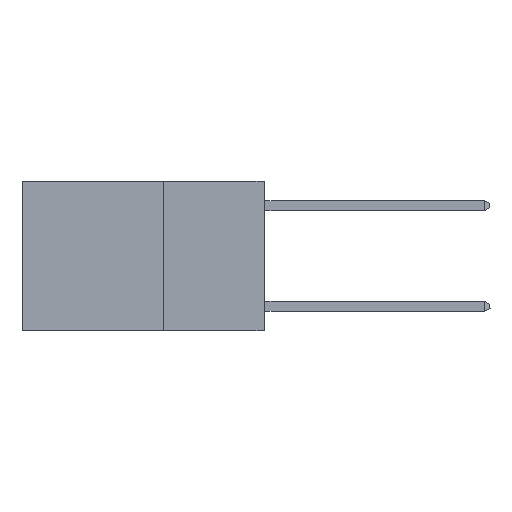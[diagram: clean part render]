
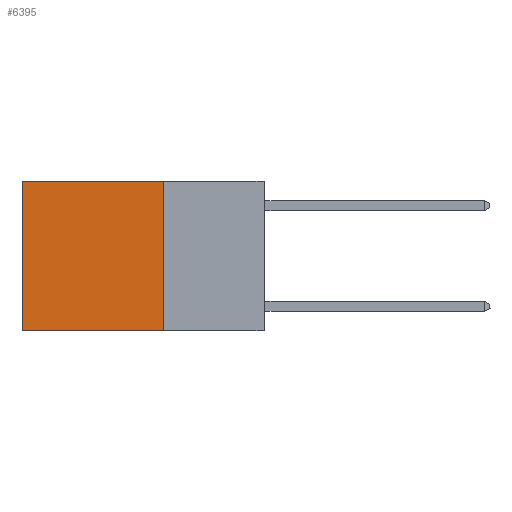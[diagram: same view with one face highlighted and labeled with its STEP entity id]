
A CAD part, left-side view. The second image highlights one B-rep face of the part: STEP entity #6395.
In plain terms, the highlighted planar face has unit normal (-1, 0, 0).
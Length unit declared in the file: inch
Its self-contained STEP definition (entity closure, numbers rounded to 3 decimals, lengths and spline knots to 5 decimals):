
#464 = CARTESIAN_POINT ( 'NONE',  ( 0.2625, 0.25, -0.37 ) ) ;
#875 = PLANE ( 'NONE',  #8818 ) ;
#888 = CARTESIAN_POINT ( 'NONE',  ( 0.2625, 0.25, -0.37 ) ) ;
#2189 = VERTEX_POINT ( 'NONE', #6380 ) ;
#2240 = DIRECTION ( 'NONE',  ( 1., 0., 0. ) ) ;
#2431 = CARTESIAN_POINT ( 'NONE',  ( 0.2625, 0.25, 0. ) ) ;
#2490 = LINE ( 'NONE', #888, #2856 ) ;
#2638 = CARTESIAN_POINT ( 'NONE',  ( 0.2625, 0.25, 0. ) ) ;
#2707 = CARTESIAN_POINT ( 'NONE',  ( 0.2625, 0.25, 0. ) ) ;
#2856 = VECTOR ( 'NONE', #7996, 39.37008 ) ;
#3342 = VERTEX_POINT ( 'NONE', #464 ) ;
#3536 = EDGE_CURVE ( 'NONE', #11224, #3342, #7976, .T. ) ;
#3630 = EDGE_LOOP ( 'NONE', ( #8910, #8903, #8497, #6399 ) ) ;
#4560 = EDGE_CURVE ( 'NONE', #11224, #5095, #10932, .T. ) ;
#4590 = DIRECTION ( 'NONE',  ( 0., 1., 0. ) ) ;
#5095 = VERTEX_POINT ( 'NONE', #8430 ) ;
#5472 = EDGE_CURVE ( 'NONE', #5095, #2189, #7646, .T. ) ;
#5748 = EDGE_CURVE ( 'NONE', #3342, #2189, #2490, .T. ) ;
#5910 = VECTOR ( 'NONE', #10448, 39.37008 ) ;
#6380 = CARTESIAN_POINT ( 'NONE',  ( 0.2625, 0.6, -0.37 ) ) ;
#6395 = ADVANCED_FACE ( 'NONE', ( #9021 ), #875, .F. ) ;
#6399 = ORIENTED_EDGE ( 'NONE', *, *, #4560, .T. ) ;
#6631 = CARTESIAN_POINT ( 'NONE',  ( 0.2625, 0.25, 0. ) ) ;
#7559 = VECTOR ( 'NONE', #8635, 39.37008 ) ;
#7646 = LINE ( 'NONE', #11299, #7559 ) ;
#7761 = VECTOR ( 'NONE', #4590, 39.37008 ) ;
#7976 = LINE ( 'NONE', #2638, #5910 ) ;
#7996 = DIRECTION ( 'NONE',  ( 0., 1., 0. ) ) ;
#8430 = CARTESIAN_POINT ( 'NONE',  ( 0.2625, 0.6, 0. ) ) ;
#8497 = ORIENTED_EDGE ( 'NONE', *, *, #3536, .F. ) ;
#8635 = DIRECTION ( 'NONE',  ( 0., 0., -1. ) ) ;
#8818 = AXIS2_PLACEMENT_3D ( 'NONE', #6631, #2240, #11043 ) ;
#8903 = ORIENTED_EDGE ( 'NONE', *, *, #5748, .F. ) ;
#8910 = ORIENTED_EDGE ( 'NONE', *, *, #5472, .T. ) ;
#9021 = FACE_OUTER_BOUND ( 'NONE', #3630, .T. ) ;
#10448 = DIRECTION ( 'NONE',  ( 0., 0., -1. ) ) ;
#10932 = LINE ( 'NONE', #2707, #7761 ) ;
#11043 = DIRECTION ( 'NONE',  ( 0., 0., -1. ) ) ;
#11224 = VERTEX_POINT ( 'NONE', #2431 ) ;
#11299 = CARTESIAN_POINT ( 'NONE',  ( 0.2625, 0.6, 0. ) ) ;
